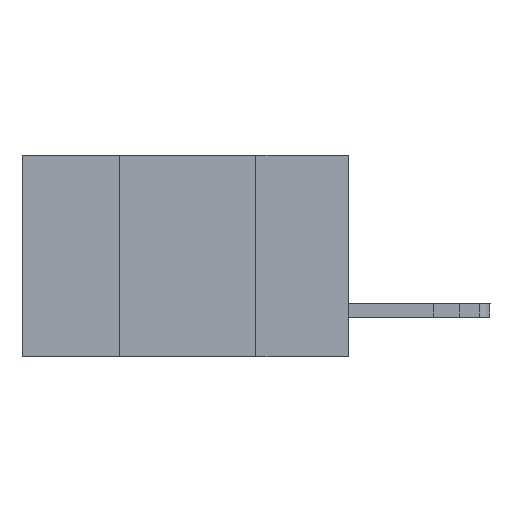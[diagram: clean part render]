
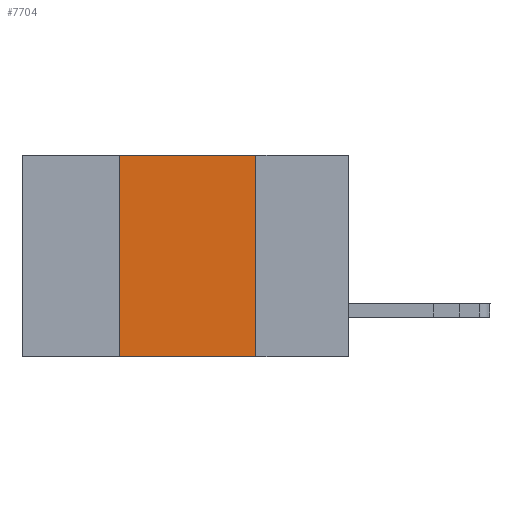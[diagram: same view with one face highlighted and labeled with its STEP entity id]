
A CAD part, left-side view. The second image highlights one B-rep face of the part: STEP entity #7704.
In plain terms, the highlighted planar face has unit normal (-1, 0, 0).
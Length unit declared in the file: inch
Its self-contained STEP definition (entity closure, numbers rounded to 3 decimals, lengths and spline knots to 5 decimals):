
#719 = DIRECTION ( 'NONE',  ( 0., 0., -1. ) ) ;
#1604 = CARTESIAN_POINT ( 'NONE',  ( 0., 0.6, -0.37 ) ) ;
#2830 = EDGE_CURVE ( 'NONE', #10574, #4530, #13110, .T. ) ;
#3065 = CARTESIAN_POINT ( 'NONE',  ( 0., 0.6, 0. ) ) ;
#3249 = EDGE_CURVE ( 'NONE', #14787, #4530, #4478, .T. ) ;
#4478 = LINE ( 'NONE', #1604, #9933 ) ;
#4530 = VERTEX_POINT ( 'NONE', #10780 ) ;
#4548 = LINE ( 'NONE', #3065, #12680 ) ;
#4581 = DIRECTION ( 'NONE',  ( 0., -1., 0. ) ) ;
#5265 = ORIENTED_EDGE ( 'NONE', *, *, #3249, .T. ) ;
#5346 = CARTESIAN_POINT ( 'NONE',  ( 0., 0.17, 0. ) ) ;
#6021 = AXIS2_PLACEMENT_3D ( 'NONE', #18467, #9407, #719 ) ;
#6039 = ORIENTED_EDGE ( 'NONE', *, *, #15262, .F. ) ;
#7585 = LINE ( 'NONE', #19426, #7989 ) ;
#7704 = ADVANCED_FACE ( 'NONE', ( #16892 ), #18768, .F. ) ;
#7989 = VECTOR ( 'NONE', #10458, 39.37008 ) ;
#8321 = ORIENTED_EDGE ( 'NONE', *, *, #9704, .F. ) ;
#9407 = DIRECTION ( 'NONE',  ( 1., 0., 0. ) ) ;
#9704 = EDGE_CURVE ( 'NONE', #14787, #16342, #7585, .T. ) ;
#9933 = VECTOR ( 'NONE', #4581, 39.37008 ) ;
#10458 = DIRECTION ( 'NONE',  ( 0., 0., 1. ) ) ;
#10574 = VERTEX_POINT ( 'NONE', #5346 ) ;
#10683 = CARTESIAN_POINT ( 'NONE',  ( 0., 0.42, -0.37 ) ) ;
#10780 = CARTESIAN_POINT ( 'NONE',  ( 0., 0.17, -0.37 ) ) ;
#12680 = VECTOR ( 'NONE', #16472, 39.37008 ) ;
#13110 = LINE ( 'NONE', #14486, #13314 ) ;
#13314 = VECTOR ( 'NONE', #15777, 39.37008 ) ;
#13495 = ORIENTED_EDGE ( 'NONE', *, *, #2830, .F. ) ;
#14486 = CARTESIAN_POINT ( 'NONE',  ( 0., 0.17, -0.37 ) ) ;
#14787 = VERTEX_POINT ( 'NONE', #10683 ) ;
#15262 = EDGE_CURVE ( 'NONE', #16342, #10574, #4548, .T. ) ;
#15777 = DIRECTION ( 'NONE',  ( 0., 0., -1. ) ) ;
#16342 = VERTEX_POINT ( 'NONE', #17798 ) ;
#16472 = DIRECTION ( 'NONE',  ( 0., -1., 0. ) ) ;
#16892 = FACE_OUTER_BOUND ( 'NONE', #17733, .T. ) ;
#17733 = EDGE_LOOP ( 'NONE', ( #13495, #6039, #8321, #5265 ) ) ;
#17798 = CARTESIAN_POINT ( 'NONE',  ( 0., 0.42, 0. ) ) ;
#18467 = CARTESIAN_POINT ( 'NONE',  ( 0., 0.6, 0. ) ) ;
#18768 = PLANE ( 'NONE',  #6021 ) ;
#19426 = CARTESIAN_POINT ( 'NONE',  ( 0., 0.42, -0.37 ) ) ;
